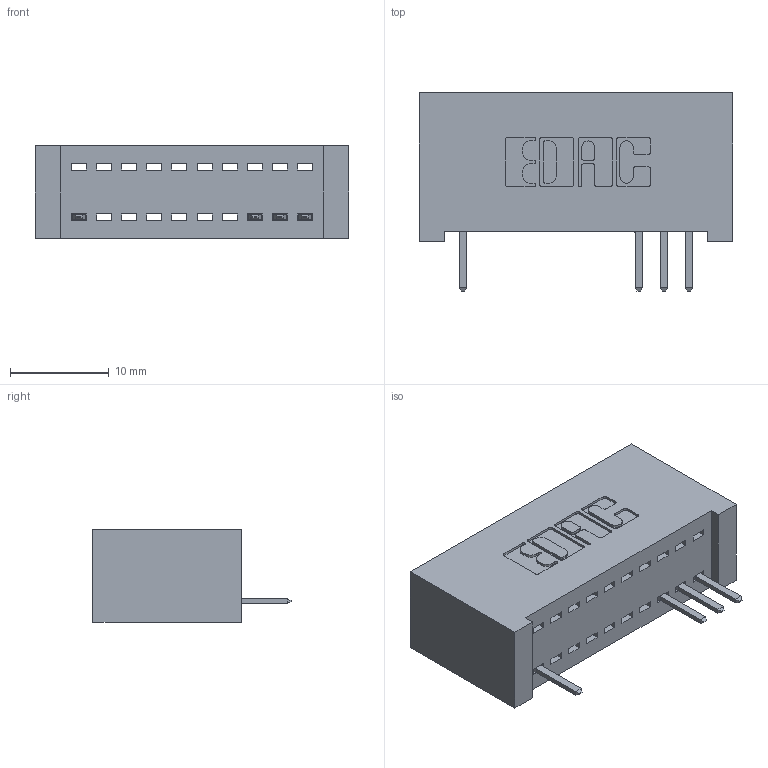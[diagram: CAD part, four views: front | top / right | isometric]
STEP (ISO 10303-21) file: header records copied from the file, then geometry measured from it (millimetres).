
FILE_DESCRIPTION (( 'STEP AP203' ), '1' );
FILE_NAME ('392-010-520-101.STEP', '2018-08-14T20:02:20', ( '' ), ( '' ), 'SwSTEP 2.0', 'SolidWorks 2016', '' );
FILE_SCHEMA (( 'CONFIG_CONTROL_DESIGN' ));
Length unit declared in the file: inch
Products named in the file (3): 342 Part_Lugless; 345-292-001_345-293-120; 392-010-520-101
Assembly tree (5 placements, depth 2):
  392-010-520-101
    342 Part_Lugless
    345-292-001_345-293-120  x4
Bounding box: 31.65 x 20.02 x 9.4 mm (x, y, z)
Volume: 2985.9 mm3; surface area: 3718.1 mm2
Topology: 5 solids, 5 shells, 422 faces, 1263 edges, 830 vertices
Faces by surface type: plane 310, cylinder 112
Entity records: 9765 total; most frequent: CARTESIAN_POINT 1734, ORIENTED_EDGE 1674, DIRECTION 1501, EDGE_CURVE 837, VECTOR 713, LINE 713, VERTEX_POINT 554, AXIS2_PLACEMENT_3D 394
